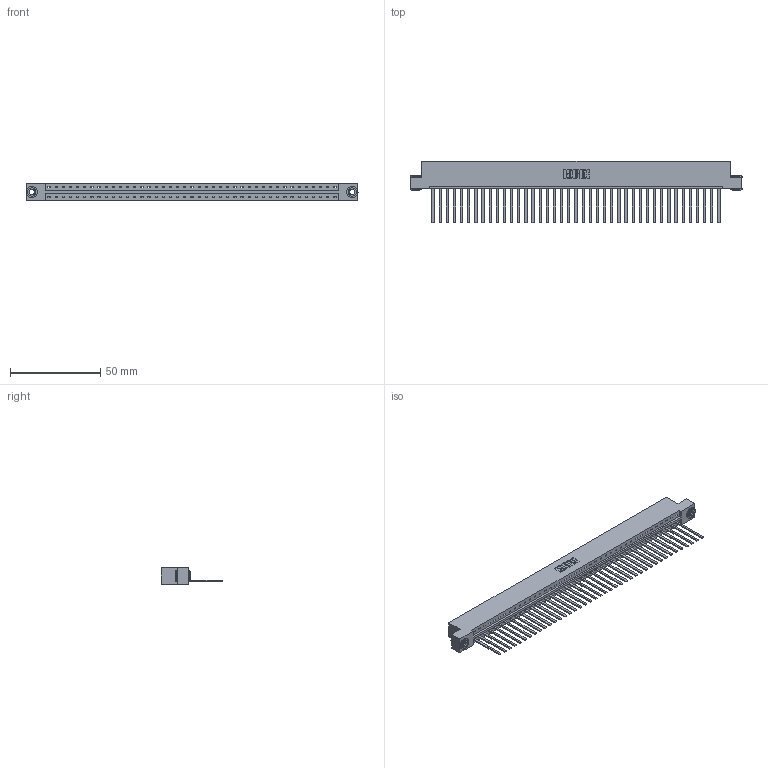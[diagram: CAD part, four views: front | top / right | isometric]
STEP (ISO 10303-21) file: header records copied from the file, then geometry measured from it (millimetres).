
FILE_DESCRIPTION (( 'STEP AP203' ), '1' );
FILE_NAME ('333-041-544-103.STEP', '2018-08-03T15:40:01', ( '' ), ( '' ), 'SwSTEP 2.0', 'SolidWorks 2016', '' );
FILE_SCHEMA (( 'CONFIG_CONTROL_DESIGN' ));
Length unit declared in the file: inch
Products named in the file (4): 333 Part_Flush - .156 Dia - TH; 345-292-001_345-293-144; 345-250-002_345-250-002-102; 333-041-544-103
Assembly tree (44 placements, depth 2):
  333-041-544-103
    333 Part_Flush - .156 Dia - TH
    345-292-001_345-293-144  x41
    345-250-002_345-250-002-102  x2
Bounding box: 184 x 34.3 x 9.4 mm (x, y, z)
Volume: 19001 mm3; surface area: 22323.8 mm2
Topology: 44 solids, 44 shells, 2284 faces, 6865 edges, 4518 vertices
Faces by surface type: plane 1638, cylinder 638, cone 8
Entity records: 25660 total; most frequent: CARTESIAN_POINT 4404, ORIENTED_EDGE 4374, DIRECTION 3747, EDGE_CURVE 2187, VECTOR 2039, LINE 2039, VERTEX_POINT 1454, AXIS2_PLACEMENT_3D 854
